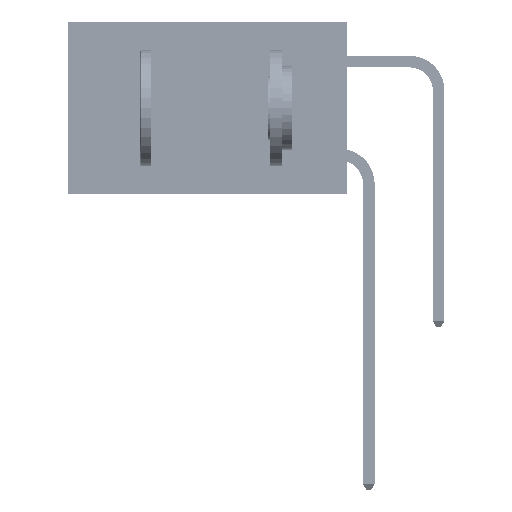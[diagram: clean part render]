
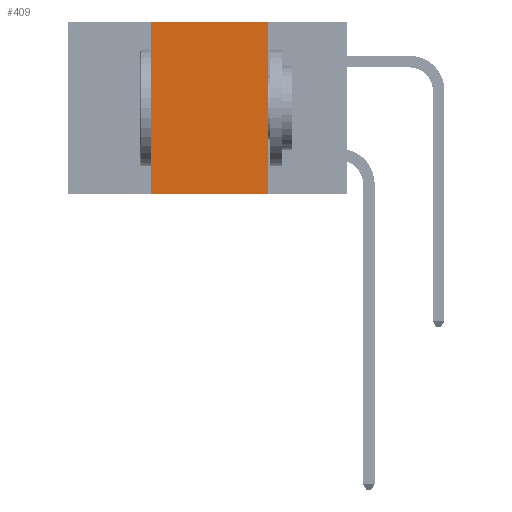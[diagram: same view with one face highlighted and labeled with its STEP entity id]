
A CAD part, left-side view. The second image highlights one B-rep face of the part: STEP entity #409.
In plain terms, the highlighted planar face has unit normal (-1, 0, 0).
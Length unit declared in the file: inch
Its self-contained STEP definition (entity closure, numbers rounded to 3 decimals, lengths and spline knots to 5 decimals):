
#409 = ADVANCED_FACE ( 'NONE', ( #48407 ), #21205, .F. ) ;
#486 = VECTOR ( 'NONE', #27330, 39.37008 ) ;
#512 = DIRECTION ( 'NONE',  ( 1., 0., 0. ) ) ;
#1776 = LINE ( 'NONE', #44270, #486 ) ;
#1974 = VECTOR ( 'NONE', #23130, 39.37008 ) ;
#3702 = AXIS2_PLACEMENT_3D ( 'NONE', #17210, #512, #29517 ) ;
#6678 = CARTESIAN_POINT ( 'NONE',  ( 0., 0.17, -0.37 ) ) ;
#7251 = LINE ( 'NONE', #9406, #37087 ) ;
#9406 = CARTESIAN_POINT ( 'NONE',  ( 0., 0.17, 0. ) ) ;
#12671 = EDGE_CURVE ( 'NONE', #51215, #41848, #7251, .T. ) ;
#13244 = LINE ( 'NONE', #16603, #23593 ) ;
#16603 = CARTESIAN_POINT ( 'NONE',  ( 0., 0.42, 0. ) ) ;
#17210 = CARTESIAN_POINT ( 'NONE',  ( 0., 0.6, 0. ) ) ;
#19508 = ORIENTED_EDGE ( 'NONE', *, *, #12671, .F. ) ;
#21205 = PLANE ( 'NONE',  #3702 ) ;
#23130 = DIRECTION ( 'NONE',  ( 0., -1., 0. ) ) ;
#23593 = VECTOR ( 'NONE', #25672, 39.37008 ) ;
#25672 = DIRECTION ( 'NONE',  ( 0., 0., 1. ) ) ;
#25932 = DIRECTION ( 'NONE',  ( 0., 0., -1. ) ) ;
#27330 = DIRECTION ( 'NONE',  ( 0., -1., 0. ) ) ;
#28790 = EDGE_CURVE ( 'NONE', #51156, #45565, #13244, .T. ) ;
#29517 = DIRECTION ( 'NONE',  ( 0., 0., -1. ) ) ;
#30224 = ORIENTED_EDGE ( 'NONE', *, *, #42706, .T. ) ;
#30547 = CARTESIAN_POINT ( 'NONE',  ( 0., 0.17, 0. ) ) ;
#31761 = CARTESIAN_POINT ( 'NONE',  ( 0., 0.6, -0.37 ) ) ;
#35020 = LINE ( 'NONE', #31761, #1974 ) ;
#37087 = VECTOR ( 'NONE', #25932, 39.37008 ) ;
#38349 = ORIENTED_EDGE ( 'NONE', *, *, #45012, .F. ) ;
#41848 = VERTEX_POINT ( 'NONE', #6678 ) ;
#42645 = CARTESIAN_POINT ( 'NONE',  ( 0., 0.42, -0.37 ) ) ;
#42706 = EDGE_CURVE ( 'NONE', #51156, #41848, #35020, .T. ) ;
#43319 = CARTESIAN_POINT ( 'NONE',  ( 0., 0.42, 0. ) ) ;
#44270 = CARTESIAN_POINT ( 'NONE',  ( 0., 0.6, 0. ) ) ;
#45012 = EDGE_CURVE ( 'NONE', #45565, #51215, #1776, .T. ) ;
#45565 = VERTEX_POINT ( 'NONE', #43319 ) ;
#47378 = EDGE_LOOP ( 'NONE', ( #19508, #38349, #48129, #30224 ) ) ;
#48129 = ORIENTED_EDGE ( 'NONE', *, *, #28790, .F. ) ;
#48407 = FACE_OUTER_BOUND ( 'NONE', #47378, .T. ) ;
#51156 = VERTEX_POINT ( 'NONE', #42645 ) ;
#51215 = VERTEX_POINT ( 'NONE', #30547 ) ;
